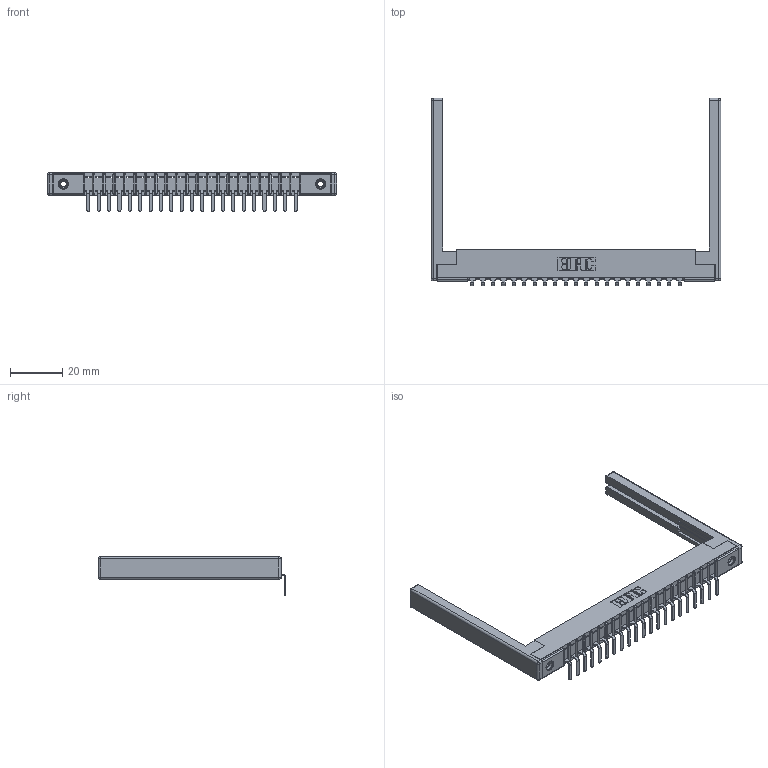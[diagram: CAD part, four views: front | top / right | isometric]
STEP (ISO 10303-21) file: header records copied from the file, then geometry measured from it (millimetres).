
FILE_DESCRIPTION (( 'STEP AP203' ), '1' );
FILE_NAME ('357-021-559-168.STEP', '2022-07-12T22:26:14', ( '' ), ( '' ), 'SwSTEP 2.0', 'SolidWorks 2020', '' );
FILE_SCHEMA (( 'CONFIG_CONTROL_DESIGN' ));
Length unit declared in the file: inch
Products named in the file (5): 307-220-068; 345-250-001_345-250-001-102; 307-290-001_558 559 - 1 (Single); 307 Part_.156 Dia Mounting Holes; 357-021-559-168
Assembly tree (26 placements, depth 2):
  357-021-559-168
    307 Part_.156 Dia Mounting Holes
    307-290-001_558 559 - 1 (Single)  x21
    307-220-068  x2
    345-250-001_345-250-001-102  x2
Bounding box: 110.64 x 71.67 x 14.81 mm (x, y, z)
Volume: 11571 mm3; surface area: 14996.7 mm2
Topology: 26 solids, 26 shells, 1554 faces, 4367 edges, 2802 vertices
Faces by surface type: plane 977, cylinder 509, sphere 52, cone 12, torus 4
Entity records: 23455 total; most frequent: CARTESIAN_POINT 3909, ORIENTED_EDGE 3884, DIRECTION 3832, EDGE_CURVE 1942, VECTOR 1478, LINE 1478, VERTEX_POINT 1254, AXIS2_PLACEMENT_3D 1177
